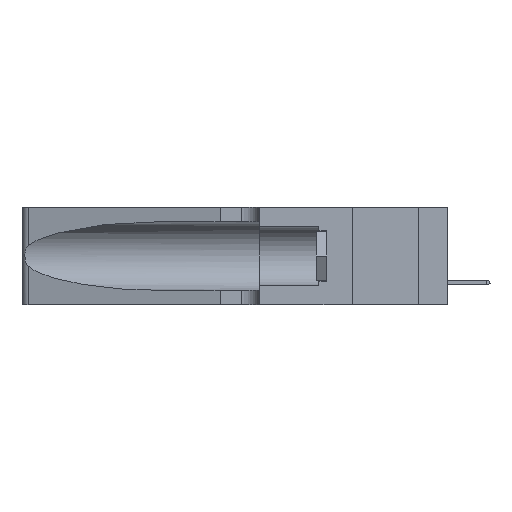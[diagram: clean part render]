
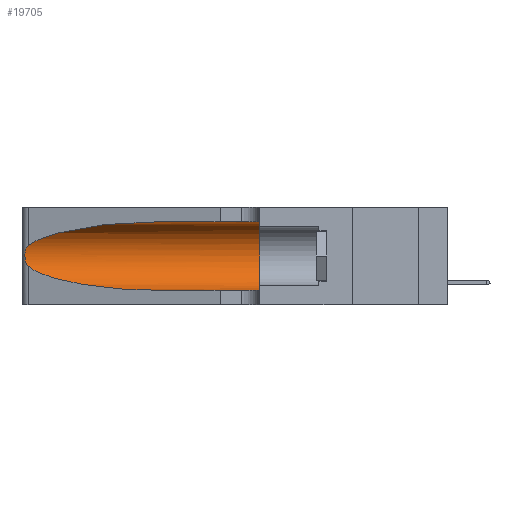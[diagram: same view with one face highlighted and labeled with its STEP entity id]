
A CAD part, left-side view. The second image highlights one B-rep face of the part: STEP entity #19705.
In plain terms, the highlighted cylindrical face has radius 3.308 mm (diameter 6.617 mm), a partial arc.
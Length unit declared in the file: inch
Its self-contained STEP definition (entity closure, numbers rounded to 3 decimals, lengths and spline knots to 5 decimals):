
#109 = CARTESIAN_POINT ( 'NONE',  ( 0.25487, 1.22718, 0.22369 ) ) ;
#354 = CIRCLE ( 'NONE', #12310, 0.13025 ) ;
#866 = CARTESIAN_POINT ( 'NONE',  ( 0.26075, 1.23896, 0.178 ) ) ;
#1036 = VERTEX_POINT ( 'NONE', #13464 ) ;
#2642 = EDGE_CURVE ( 'NONE', #7038, #5884, #12328, .T. ) ;
#2728 = FACE_OUTER_BOUND ( 'NONE', #19590, .T. ) ;
#3438 = CARTESIAN_POINT ( 'NONE',  ( 0.1305, 0.35, 0.05475 ) ) ;
#3447 = CARTESIAN_POINT ( 'NONE',  ( 0.25856, 1.23593, 0.16098 ) ) ;
#4632 = CARTESIAN_POINT ( 'NONE',  ( 0.25639, 1.23184, 0.21858 ) ) ;
#5636 = CARTESIAN_POINT ( 'NONE',  ( 0.25487, 1.22718, 0.22369 ) ) ;
#5884 = VERTEX_POINT ( 'NONE', #9958 ) ;
#6596 = CARTESIAN_POINT ( 'NONE',  ( 0.26017, 1.23833, 0.17102 ) ) ;
#7002 = CARTESIAN_POINT ( 'NONE',  ( 0.1305, 0.72297, 0.05475 ) ) ;
#7038 = VERTEX_POINT ( 'NONE', #7246 ) ;
#7077 = CARTESIAN_POINT ( 'NONE',  ( 0.25487, 1.22718, 0.14631 ) ) ;
#7184 = CARTESIAN_POINT ( 'NONE',  ( 0.1305, 0.35, 0.185 ) ) ;
#7246 = CARTESIAN_POINT ( 'NONE',  ( 0.25487, 1.22718, 0.14631 ) ) ;
#7263 = CARTESIAN_POINT ( 'NONE',  ( 0.25487, 1.22718, 0.14631 ) ) ;
#7365 = DIRECTION ( 'NONE',  ( 0., 0., -1. ) ) ;
#7919 = ORIENTED_EDGE ( 'NONE', *, *, #21697, .F. ) ;
#8256 = LINE ( 'NONE', #22081, #12709 ) ;
#8261 = EDGE_CURVE ( 'NONE', #21384, #9912, #19405, .T. ) ;
#8436 = CARTESIAN_POINT ( 'NONE',  ( 0.26018, 1.23835, 0.19895 ) ) ;
#8928 = LINE ( 'NONE', #15494, #17906 ) ;
#8944 = DIRECTION ( 'NONE',  ( 0., 1., 0. ) ) ;
#9027 = CARTESIAN_POINT ( 'NONE',  ( 0.18966, 0.96281, 0.05475 ) ) ;
#9260 = B_SPLINE_CURVE_WITH_KNOTS ( 'NONE', 3,
 ( #19804, #12185, #4632, #21739, #19885, #8436, #12271, #866, #6596, #3447, #16447, #24360, #22476, #7077 ),
 .UNSPECIFIED., .F., .F.,
 ( 4, 2, 2, 2, 2, 2, 4 ),
 ( 0., 0.00027, 0.00053, 0.00107, 0.0016, 0.00187, 0.00214 ),
 .UNSPECIFIED. ) ;
#9285 = CARTESIAN_POINT ( 'NONE',  ( 0.2373, 1.15595, 0.28018 ) ) ;
#9912 = VERTEX_POINT ( 'NONE', #109 ) ;
#9958 = CARTESIAN_POINT ( 'NONE',  ( 0.1305, 0.72297, 0.05475 ) ) ;
#10493 = EDGE_CURVE ( 'NONE', #9912, #7038, #9260, .T. ) ;
#10733 = CYLINDRICAL_SURFACE ( 'NONE', #15224, 0.13025 ) ;
#11322 = ORIENTED_EDGE ( 'NONE', *, *, #11513, .T. ) ;
#11392 = VERTEX_POINT ( 'NONE', #3438 ) ;
#11513 = EDGE_CURVE ( 'NONE', #5884, #11392, #8928, .T. ) ;
#11608 = DIRECTION ( 'NONE',  ( 0., -1., 0. ) ) ;
#12185 = CARTESIAN_POINT ( 'NONE',  ( 0.25555, 1.22994, 0.2215 ) ) ;
#12271 = CARTESIAN_POINT ( 'NONE',  ( 0.26075, 1.23896, 0.19203 ) ) ;
#12310 = AXIS2_PLACEMENT_3D ( 'NONE', #7184, #8944, #24058 ) ;
#12328 =( BOUNDED_CURVE ( )  B_SPLINE_CURVE ( 3, ( #7263, #18641, #9027, #7002 ),
 .UNSPECIFIED., .F., .F. ) 
 B_SPLINE_CURVE_WITH_KNOTS ( ( 4, 4 ),
 ( 3.44316, 4.71239 ),
 .UNSPECIFIED. ) 
 CURVE ( )  GEOMETRIC_REPRESENTATION_ITEM ( )  RATIONAL_B_SPLINE_CURVE ( ( 1., 0.87, 0.87, 1. ) ) 
 REPRESENTATION_ITEM ( '' )  );
#12709 = VECTOR ( 'NONE', #21835, 39.37008 ) ;
#13464 = CARTESIAN_POINT ( 'NONE',  ( 0.1305, 0.35, 0.31525 ) ) ;
#14957 = CARTESIAN_POINT ( 'NONE',  ( 0.1305, 0.72297, 0.31525 ) ) ;
#15224 = AXIS2_PLACEMENT_3D ( 'NONE', #20485, #18655, #7365 ) ;
#15494 = CARTESIAN_POINT ( 'NONE',  ( 0.1305, 1.61858, 0.05475 ) ) ;
#15841 = ORIENTED_EDGE ( 'NONE', *, *, #8261, .T. ) ;
#16447 = CARTESIAN_POINT ( 'NONE',  ( 0.25789, 1.23486, 0.15765 ) ) ;
#16452 = ORIENTED_EDGE ( 'NONE', *, *, #17874, .F. ) ;
#16896 = CARTESIAN_POINT ( 'NONE',  ( 0.18966, 0.96281, 0.31525 ) ) ;
#17336 = ORIENTED_EDGE ( 'NONE', *, *, #10493, .T. ) ;
#17874 = EDGE_CURVE ( 'NONE', #1036, #11392, #354, .T. ) ;
#17906 = VECTOR ( 'NONE', #11608, 39.37008 ) ;
#18478 = ORIENTED_EDGE ( 'NONE', *, *, #2642, .T. ) ;
#18641 = CARTESIAN_POINT ( 'NONE',  ( 0.2373, 1.15595, 0.08982 ) ) ;
#18655 = DIRECTION ( 'NONE',  ( 0., -1., 0. ) ) ;
#19405 =( BOUNDED_CURVE ( )  B_SPLINE_CURVE ( 3, ( #14957, #16896, #9285, #5636 ),
 .UNSPECIFIED., .F., .F. ) 
 B_SPLINE_CURVE_WITH_KNOTS ( ( 4, 4 ),
 ( 1.5708, 2.84003 ),
 .UNSPECIFIED. ) 
 CURVE ( )  GEOMETRIC_REPRESENTATION_ITEM ( )  RATIONAL_B_SPLINE_CURVE ( ( 1., 0.87, 0.87, 1. ) ) 
 REPRESENTATION_ITEM ( '' )  );
#19590 = EDGE_LOOP ( 'NONE', ( #15841, #17336, #18478, #11322, #16452, #7919 ) ) ;
#19705 = ADVANCED_FACE ( 'NONE', ( #2728 ), #10733, .F. ) ;
#19804 = CARTESIAN_POINT ( 'NONE',  ( 0.25487, 1.22718, 0.22369 ) ) ;
#19885 = CARTESIAN_POINT ( 'NONE',  ( 0.25854, 1.2359, 0.20912 ) ) ;
#20485 = CARTESIAN_POINT ( 'NONE',  ( 0.1305, 1.61858, 0.185 ) ) ;
#21384 = VERTEX_POINT ( 'NONE', #23186 ) ;
#21697 = EDGE_CURVE ( 'NONE', #21384, #1036, #8256, .T. ) ;
#21739 = CARTESIAN_POINT ( 'NONE',  ( 0.25787, 1.23484, 0.2124 ) ) ;
#21835 = DIRECTION ( 'NONE',  ( 0., -1., 0. ) ) ;
#22081 = CARTESIAN_POINT ( 'NONE',  ( 0.1305, 1.61858, 0.31525 ) ) ;
#22476 = CARTESIAN_POINT ( 'NONE',  ( 0.25555, 1.22993, 0.14849 ) ) ;
#23186 = CARTESIAN_POINT ( 'NONE',  ( 0.1305, 0.72297, 0.31525 ) ) ;
#24058 = DIRECTION ( 'NONE',  ( 0., 0., 1. ) ) ;
#24360 = CARTESIAN_POINT ( 'NONE',  ( 0.25639, 1.23186, 0.15144 ) ) ;
